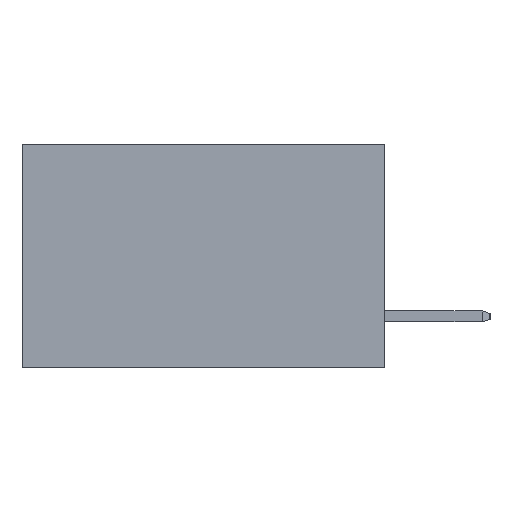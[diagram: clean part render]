
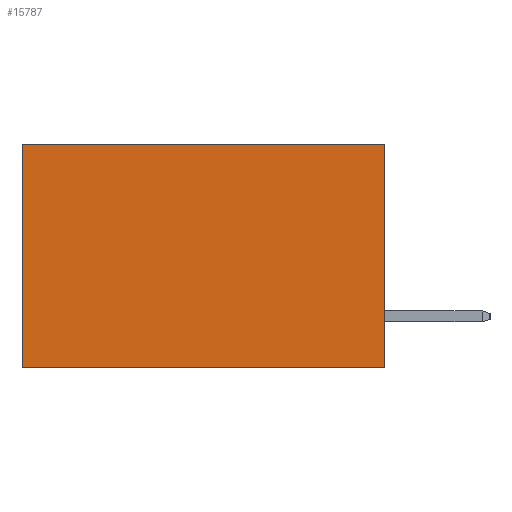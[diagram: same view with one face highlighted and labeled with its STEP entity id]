
A CAD part, left-side view. The second image highlights one B-rep face of the part: STEP entity #15787.
In plain terms, the highlighted planar face has unit normal (-1, 0, 0).
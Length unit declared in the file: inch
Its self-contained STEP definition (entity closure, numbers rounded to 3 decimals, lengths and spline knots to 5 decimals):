
#475 = CARTESIAN_POINT ( 'NONE',  ( 0.2615, 0.6, 0. ) ) ;
#1081 = CARTESIAN_POINT ( 'NONE',  ( 0.2615, 0., -0.37 ) ) ;
#1450 = CARTESIAN_POINT ( 'NONE',  ( 0.2615, 0., 0. ) ) ;
#1496 = DIRECTION ( 'NONE',  ( 0., 1., 0. ) ) ;
#1569 = LINE ( 'NONE', #8957, #15786 ) ;
#1701 = DIRECTION ( 'NONE',  ( 0., 1., 0. ) ) ;
#1946 = EDGE_LOOP ( 'NONE', ( #13301, #11068, #9949, #15517 ) ) ;
#2275 = EDGE_CURVE ( 'NONE', #14655, #17530, #3814, .T. ) ;
#2855 = DIRECTION ( 'NONE',  ( 0., 0., -1. ) ) ;
#3814 = LINE ( 'NONE', #8869, #11009 ) ;
#4027 = CARTESIAN_POINT ( 'NONE',  ( 0.2615, 0., -0.37 ) ) ;
#4100 = EDGE_CURVE ( 'NONE', #14655, #13634, #7395, .T. ) ;
#4319 = EDGE_CURVE ( 'NONE', #13634, #17760, #10095, .T. ) ;
#5555 = PLANE ( 'NONE',  #14223 ) ;
#5811 = VECTOR ( 'NONE', #12228, 39.37008 ) ;
#5899 = CARTESIAN_POINT ( 'NONE',  ( 0.2615, 0.6, -0.37 ) ) ;
#5959 = CARTESIAN_POINT ( 'NONE',  ( 0.2615, 0., 0. ) ) ;
#6967 = DIRECTION ( 'NONE',  ( 0., 0., -1. ) ) ;
#7395 = LINE ( 'NONE', #1450, #10338 ) ;
#8869 = CARTESIAN_POINT ( 'NONE',  ( 0.2615, 0., -0.37 ) ) ;
#8957 = CARTESIAN_POINT ( 'NONE',  ( 0.2615, 0., -0.37 ) ) ;
#9949 = ORIENTED_EDGE ( 'NONE', *, *, #2275, .F. ) ;
#10095 = LINE ( 'NONE', #13041, #5811 ) ;
#10338 = VECTOR ( 'NONE', #1496, 39.37008 ) ;
#11009 = VECTOR ( 'NONE', #2855, 39.37008 ) ;
#11068 = ORIENTED_EDGE ( 'NONE', *, *, #14692, .F. ) ;
#12228 = DIRECTION ( 'NONE',  ( 0., 0., -1. ) ) ;
#13041 = CARTESIAN_POINT ( 'NONE',  ( 0.2615, 0.6, -0.37 ) ) ;
#13301 = ORIENTED_EDGE ( 'NONE', *, *, #4319, .T. ) ;
#13634 = VERTEX_POINT ( 'NONE', #475 ) ;
#14223 = AXIS2_PLACEMENT_3D ( 'NONE', #1081, #15422, #6967 ) ;
#14655 = VERTEX_POINT ( 'NONE', #5959 ) ;
#14692 = EDGE_CURVE ( 'NONE', #17530, #17760, #1569, .T. ) ;
#14856 = FACE_OUTER_BOUND ( 'NONE', #1946, .T. ) ;
#15422 = DIRECTION ( 'NONE',  ( 1., 0., 0. ) ) ;
#15517 = ORIENTED_EDGE ( 'NONE', *, *, #4100, .T. ) ;
#15786 = VECTOR ( 'NONE', #1701, 39.37008 ) ;
#15787 = ADVANCED_FACE ( 'NONE', ( #14856 ), #5555, .F. ) ;
#17530 = VERTEX_POINT ( 'NONE', #4027 ) ;
#17760 = VERTEX_POINT ( 'NONE', #5899 ) ;
